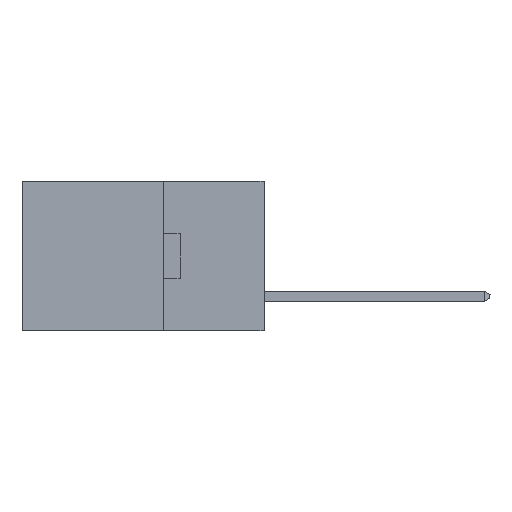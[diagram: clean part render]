
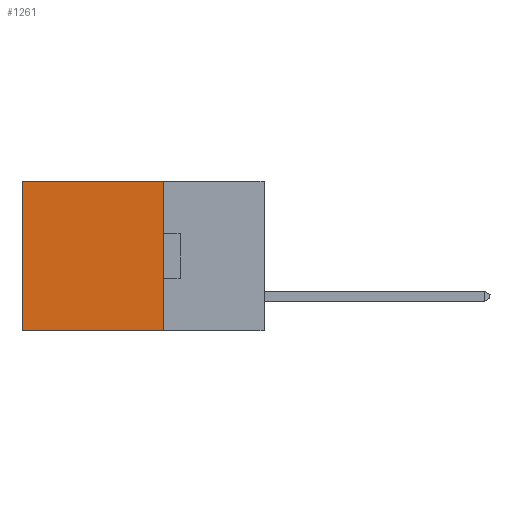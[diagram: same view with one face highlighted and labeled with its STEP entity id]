
A CAD part, left-side view. The second image highlights one B-rep face of the part: STEP entity #1261.
In plain terms, the highlighted planar face has unit normal (-1, 0, 0).
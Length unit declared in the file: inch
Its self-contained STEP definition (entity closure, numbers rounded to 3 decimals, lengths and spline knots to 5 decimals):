
#1261 = ADVANCED_FACE ( 'NONE', ( #2046 ), #10179, .F. ) ;
#1377 = VERTEX_POINT ( 'NONE', #14848 ) ;
#1837 = EDGE_CURVE ( 'NONE', #5244, #8653, #16826, .T. ) ;
#2046 = FACE_OUTER_BOUND ( 'NONE', #25447, .T. ) ;
#2274 = DIRECTION ( 'NONE',  ( 0., 0., -1. ) ) ;
#2339 = LINE ( 'NONE', #12750, #18754 ) ;
#2561 = ORIENTED_EDGE ( 'NONE', *, *, #16078, .T. ) ;
#2859 = VERTEX_POINT ( 'NONE', #25292 ) ;
#2954 = VECTOR ( 'NONE', #13764, 39.37008 ) ;
#3435 = VECTOR ( 'NONE', #2274, 39.37008 ) ;
#3734 = CARTESIAN_POINT ( 'NONE',  ( 0.2615, 0.25, 0. ) ) ;
#5244 = VERTEX_POINT ( 'NONE', #14140 ) ;
#5617 = LINE ( 'NONE', #3734, #2954 ) ;
#5904 = ORIENTED_EDGE ( 'NONE', *, *, #22519, .T. ) ;
#8611 = DIRECTION ( 'NONE',  ( 0., 0., -1. ) ) ;
#8653 = VERTEX_POINT ( 'NONE', #14783 ) ;
#10179 = PLANE ( 'NONE',  #15115 ) ;
#11510 = ORIENTED_EDGE ( 'NONE', *, *, #16154, .F. ) ;
#12562 = CARTESIAN_POINT ( 'NONE',  ( 0.2615, 0.25, -0.37 ) ) ;
#12750 = CARTESIAN_POINT ( 'NONE',  ( 0.2615, 0.6, -0.37 ) ) ;
#12885 = CARTESIAN_POINT ( 'NONE',  ( 0.2615, 0.25, -0.37 ) ) ;
#13764 = DIRECTION ( 'NONE',  ( 0., 1., 0. ) ) ;
#14140 = CARTESIAN_POINT ( 'NONE',  ( 0.2615, 0.25, 0. ) ) ;
#14783 = CARTESIAN_POINT ( 'NONE',  ( 0.2615, 0.25, -0.37 ) ) ;
#14848 = CARTESIAN_POINT ( 'NONE',  ( 0.2615, 0.6, -0.37 ) ) ;
#14877 = LINE ( 'NONE', #12885, #15783 ) ;
#15115 = AXIS2_PLACEMENT_3D ( 'NONE', #21826, #26241, #18335 ) ;
#15291 = DIRECTION ( 'NONE',  ( 0., 1., 0. ) ) ;
#15783 = VECTOR ( 'NONE', #15291, 39.37008 ) ;
#16078 = EDGE_CURVE ( 'NONE', #2859, #1377, #2339, .T. ) ;
#16154 = EDGE_CURVE ( 'NONE', #8653, #1377, #14877, .T. ) ;
#16558 = ORIENTED_EDGE ( 'NONE', *, *, #1837, .F. ) ;
#16826 = LINE ( 'NONE', #12562, #3435 ) ;
#18335 = DIRECTION ( 'NONE',  ( 0., 0., -1. ) ) ;
#18754 = VECTOR ( 'NONE', #8611, 39.37008 ) ;
#21826 = CARTESIAN_POINT ( 'NONE',  ( 0.2615, 0.25, -0.37 ) ) ;
#22519 = EDGE_CURVE ( 'NONE', #5244, #2859, #5617, .T. ) ;
#25292 = CARTESIAN_POINT ( 'NONE',  ( 0.2615, 0.6, 0. ) ) ;
#25447 = EDGE_LOOP ( 'NONE', ( #2561, #11510, #16558, #5904 ) ) ;
#26241 = DIRECTION ( 'NONE',  ( 1., 0., 0. ) ) ;
